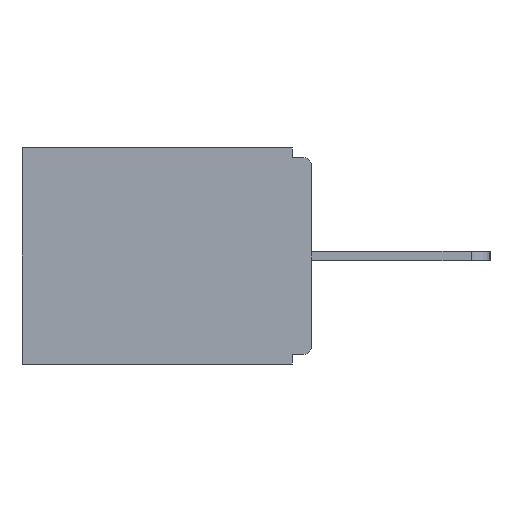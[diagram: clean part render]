
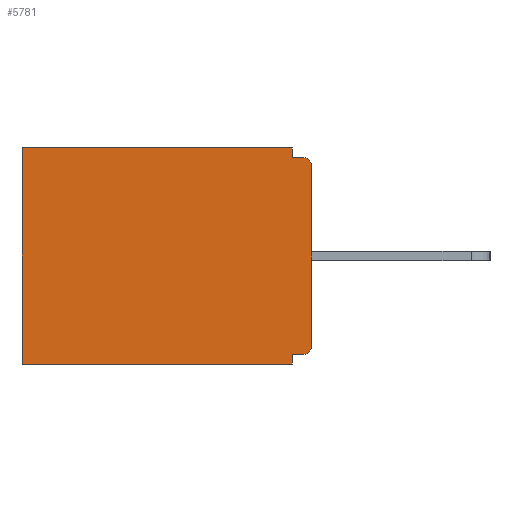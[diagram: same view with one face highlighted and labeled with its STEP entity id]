
A CAD part, left-side view. The second image highlights one B-rep face of the part: STEP entity #5781.
In plain terms, the highlighted planar face has unit normal (-1, 0, 0).
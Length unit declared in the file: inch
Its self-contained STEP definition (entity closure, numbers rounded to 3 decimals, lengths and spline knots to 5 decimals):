
#316 = DIRECTION ( 'NONE',  ( 0., 1., 0. ) ) ;
#334 = DIRECTION ( 'NONE',  ( 0., 0., -1. ) ) ;
#355 = EDGE_CURVE ( 'NONE', #2323, #14124, #19633, .T. ) ;
#564 = DIRECTION ( 'NONE',  ( 0., 1., 0. ) ) ;
#666 = EDGE_CURVE ( 'NONE', #12257, #24120, #12923, .T. ) ;
#2323 = VERTEX_POINT ( 'NONE', #19013 ) ;
#3421 = ORIENTED_EDGE ( 'NONE', *, *, #20717, .T. ) ;
#3520 = VERTEX_POINT ( 'NONE', #17698 ) ;
#3568 = CARTESIAN_POINT ( 'NONE',  ( 0.298, 0., -0.313 ) ) ;
#3729 = ORIENTED_EDGE ( 'NONE', *, *, #355, .T. ) ;
#3759 = CIRCLE ( 'NONE', #17607, 0.015 ) ;
#3777 = VERTEX_POINT ( 'NONE', #13772 ) ;
#4555 = CARTESIAN_POINT ( 'NONE',  ( 0.298, 0.015, -0.015 ) ) ;
#5006 = ORIENTED_EDGE ( 'NONE', *, *, #21519, .F. ) ;
#5348 = DIRECTION ( 'NONE',  ( 1., 0., 0. ) ) ;
#5781 = ADVANCED_FACE ( 'NONE', ( #12097 ), #6164, .F. ) ;
#6164 = PLANE ( 'NONE',  #8691 ) ;
#6448 = LINE ( 'NONE', #23854, #16056 ) ;
#6690 = VECTOR ( 'NONE', #316, 39.37008 ) ;
#6968 = VERTEX_POINT ( 'NONE', #19832 ) ;
#8211 = LINE ( 'NONE', #18556, #22927 ) ;
#8543 = CARTESIAN_POINT ( 'NONE',  ( 0.298, 0.46, 0. ) ) ;
#8632 = EDGE_CURVE ( 'NONE', #3777, #14438, #19669, .T. ) ;
#8691 = AXIS2_PLACEMENT_3D ( 'NONE', #24078, #5348, #18300 ) ;
#8907 = DIRECTION ( 'NONE',  ( 0., 0., -1. ) ) ;
#9147 = VECTOR ( 'NONE', #564, 39.37008 ) ;
#9225 = AXIS2_PLACEMENT_3D ( 'NONE', #17730, #18104, #11186 ) ;
#9990 = VECTOR ( 'NONE', #9992, 39.37008 ) ;
#9992 = DIRECTION ( 'NONE',  ( 0., -1., 0. ) ) ;
#10859 = ORIENTED_EDGE ( 'NONE', *, *, #15039, .F. ) ;
#11186 = DIRECTION ( 'NONE',  ( 0., 0., -1. ) ) ;
#11190 = DIRECTION ( 'NONE',  ( 0., 1., 0. ) ) ;
#11473 = CARTESIAN_POINT ( 'NONE',  ( 0.298, 0.015, -0.03 ) ) ;
#11538 = CARTESIAN_POINT ( 'NONE',  ( 0.298, 0., -0.03 ) ) ;
#12034 = VERTEX_POINT ( 'NONE', #11538 ) ;
#12097 = FACE_OUTER_BOUND ( 'NONE', #24757, .T. ) ;
#12257 = VERTEX_POINT ( 'NONE', #8543 ) ;
#12338 = CARTESIAN_POINT ( 'NONE',  ( 0.298, 0., -0.343 ) ) ;
#12733 = EDGE_CURVE ( 'NONE', #21602, #3520, #6448, .T. ) ;
#12923 = LINE ( 'NONE', #18068, #17448 ) ;
#13400 = DIRECTION ( 'NONE',  ( 0., 0., -1. ) ) ;
#13753 = ORIENTED_EDGE ( 'NONE', *, *, #12733, .F. ) ;
#13772 = CARTESIAN_POINT ( 'NONE',  ( 0.298, 0.031, -0.015 ) ) ;
#14124 = VERTEX_POINT ( 'NONE', #3568 ) ;
#14283 = ORIENTED_EDGE ( 'NONE', *, *, #18340, .T. ) ;
#14438 = VERTEX_POINT ( 'NONE', #4555 ) ;
#14724 = VECTOR ( 'NONE', #23956, 39.37008 ) ;
#15039 = EDGE_CURVE ( 'NONE', #2323, #21602, #19419, .T. ) ;
#15352 = LINE ( 'NONE', #20144, #14724 ) ;
#16056 = VECTOR ( 'NONE', #334, 39.37008 ) ;
#16116 = ORIENTED_EDGE ( 'NONE', *, *, #20377, .F. ) ;
#17016 = ORIENTED_EDGE ( 'NONE', *, *, #666, .T. ) ;
#17044 = VECTOR ( 'NONE', #11190, 39.37008 ) ;
#17448 = VECTOR ( 'NONE', #17806, 39.37008 ) ;
#17607 = AXIS2_PLACEMENT_3D ( 'NONE', #11473, #24886, #13400 ) ;
#17673 = LINE ( 'NONE', #18905, #17044 ) ;
#17698 = CARTESIAN_POINT ( 'NONE',  ( 0.298, 0.031, -0.343 ) ) ;
#17730 = CARTESIAN_POINT ( 'NONE',  ( 0.298, 0.015, -0.313 ) ) ;
#17806 = DIRECTION ( 'NONE',  ( 0., 0., -1. ) ) ;
#17918 = CARTESIAN_POINT ( 'NONE',  ( 0.298, 0.46, -0.343 ) ) ;
#18068 = CARTESIAN_POINT ( 'NONE',  ( 0.298, 0.46, 0. ) ) ;
#18104 = DIRECTION ( 'NONE',  ( -1., 0., 0. ) ) ;
#18300 = DIRECTION ( 'NONE',  ( 0., 0., -1. ) ) ;
#18340 = EDGE_CURVE ( 'NONE', #6968, #12257, #17673, .T. ) ;
#18373 = CARTESIAN_POINT ( 'NONE',  ( 0.298, 0., -0.328 ) ) ;
#18556 = CARTESIAN_POINT ( 'NONE',  ( 0.298, 0.031, -0.343 ) ) ;
#18905 = CARTESIAN_POINT ( 'NONE',  ( 0.298, 0., 0. ) ) ;
#19013 = CARTESIAN_POINT ( 'NONE',  ( 0.298, 0.015, -0.328 ) ) ;
#19392 = CARTESIAN_POINT ( 'NONE',  ( 0.298, 0., -0.015 ) ) ;
#19414 = ORIENTED_EDGE ( 'NONE', *, *, #20526, .F. ) ;
#19419 = LINE ( 'NONE', #18373, #9147 ) ;
#19633 = CIRCLE ( 'NONE', #9225, 0.015 ) ;
#19669 = LINE ( 'NONE', #19392, #9990 ) ;
#19832 = CARTESIAN_POINT ( 'NONE',  ( 0.298, 0.031, 0. ) ) ;
#20144 = CARTESIAN_POINT ( 'NONE',  ( 0.298, 0., 0. ) ) ;
#20377 = EDGE_CURVE ( 'NONE', #3520, #24120, #21453, .T. ) ;
#20526 = EDGE_CURVE ( 'NONE', #6968, #3777, #8211, .T. ) ;
#20570 = ORIENTED_EDGE ( 'NONE', *, *, #8632, .F. ) ;
#20717 = EDGE_CURVE ( 'NONE', #12034, #14438, #3759, .T. ) ;
#21453 = LINE ( 'NONE', #12338, #6690 ) ;
#21519 = EDGE_CURVE ( 'NONE', #12034, #14124, #15352, .T. ) ;
#21602 = VERTEX_POINT ( 'NONE', #24189 ) ;
#22927 = VECTOR ( 'NONE', #8907, 39.37008 ) ;
#23854 = CARTESIAN_POINT ( 'NONE',  ( 0.298, 0.031, -0.343 ) ) ;
#23956 = DIRECTION ( 'NONE',  ( 0., 0., -1. ) ) ;
#24078 = CARTESIAN_POINT ( 'NONE',  ( 0.298, 0., 0. ) ) ;
#24120 = VERTEX_POINT ( 'NONE', #17918 ) ;
#24189 = CARTESIAN_POINT ( 'NONE',  ( 0.298, 0.031, -0.328 ) ) ;
#24757 = EDGE_LOOP ( 'NONE', ( #3421, #20570, #19414, #14283, #17016, #16116, #13753, #10859, #3729, #5006 ) ) ;
#24886 = DIRECTION ( 'NONE',  ( -1., 0., 0. ) ) ;
